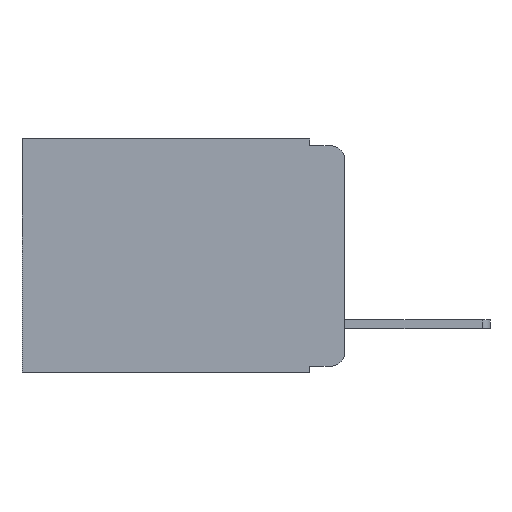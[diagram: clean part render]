
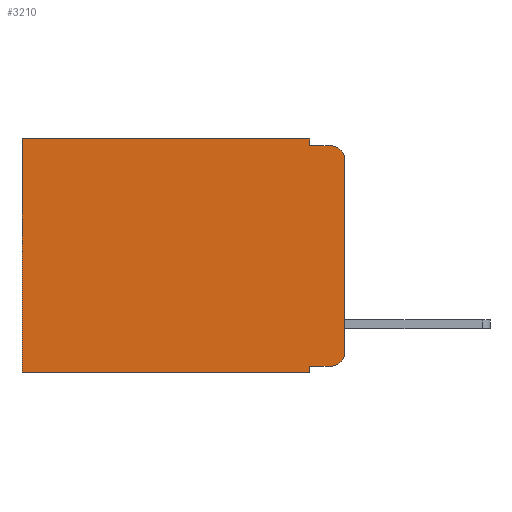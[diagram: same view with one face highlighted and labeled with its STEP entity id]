
A CAD part, left-side view. The second image highlights one B-rep face of the part: STEP entity #3210.
In plain terms, the highlighted planar face has unit normal (-1, 0, 0).
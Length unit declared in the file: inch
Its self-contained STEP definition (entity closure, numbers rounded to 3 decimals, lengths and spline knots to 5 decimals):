
#329 = ORIENTED_EDGE ( 'NONE', *, *, #6118, .T. ) ;
#747 = VERTEX_POINT ( 'NONE', #6597 ) ;
#798 = ORIENTED_EDGE ( 'NONE', *, *, #7005, .F. ) ;
#981 = DIRECTION ( 'NONE',  ( 0., 0., -1. ) ) ;
#1131 = LINE ( 'NONE', #3052, #11477 ) ;
#1171 = VERTEX_POINT ( 'NONE', #14665 ) ;
#1192 = DIRECTION ( 'NONE',  ( 0., 0., -1. ) ) ;
#1352 = DIRECTION ( 'NONE',  ( 0., 1., 0. ) ) ;
#1568 = VECTOR ( 'NONE', #981, 39.37008 ) ;
#1901 = VECTOR ( 'NONE', #5863, 39.37008 ) ;
#1966 = DIRECTION ( 'NONE',  ( -1., 0., 0. ) ) ;
#2011 = LINE ( 'NONE', #13183, #1568 ) ;
#2070 = DIRECTION ( 'NONE',  ( 0., -1., 0. ) ) ;
#2129 = CARTESIAN_POINT ( 'NONE',  ( 0.298, 0.02, -0.03 ) ) ;
#2144 = CARTESIAN_POINT ( 'NONE',  ( 0.298, 0.473, -0.343 ) ) ;
#2473 = VECTOR ( 'NONE', #2070, 39.37008 ) ;
#2561 = VERTEX_POINT ( 'NONE', #9913 ) ;
#2797 = DIRECTION ( 'NONE',  ( 0., -1., 0. ) ) ;
#3052 = CARTESIAN_POINT ( 'NONE',  ( 0.298, 0.051, 0. ) ) ;
#3210 = ADVANCED_FACE ( 'NONE', ( #14722 ), #9632, .F. ) ;
#3303 = CARTESIAN_POINT ( 'NONE',  ( 0.298, 0.02, -0.313 ) ) ;
#3344 = EDGE_CURVE ( 'NONE', #9361, #1171, #15693, .T. ) ;
#3514 = DIRECTION ( 'NONE',  ( 0., 0., -1. ) ) ;
#4251 = EDGE_CURVE ( 'NONE', #2561, #1171, #12303, .T. ) ;
#4436 = AXIS2_PLACEMENT_3D ( 'NONE', #2129, #1966, #3514 ) ;
#4647 = VERTEX_POINT ( 'NONE', #9723 ) ;
#4684 = DIRECTION ( 'NONE',  ( 0., 0., -1. ) ) ;
#5188 = EDGE_CURVE ( 'NONE', #12633, #2561, #1131, .T. ) ;
#5487 = VECTOR ( 'NONE', #7988, 39.37008 ) ;
#5863 = DIRECTION ( 'NONE',  ( 0., 0., -1. ) ) ;
#6118 = EDGE_CURVE ( 'NONE', #11728, #15267, #15860, .T. ) ;
#6186 = DIRECTION ( 'NONE',  ( 0., 0., -1. ) ) ;
#6189 = DIRECTION ( 'NONE',  ( 1., 0., 0. ) ) ;
#6198 = CARTESIAN_POINT ( 'NONE',  ( 0.298, 0.473, 0. ) ) ;
#6597 = CARTESIAN_POINT ( 'NONE',  ( 0.298, 0., -0.313 ) ) ;
#6918 = CARTESIAN_POINT ( 'NONE',  ( 0.298, 0.473, 0. ) ) ;
#7005 = EDGE_CURVE ( 'NONE', #10765, #13505, #2011, .T. ) ;
#7257 = ORIENTED_EDGE ( 'NONE', *, *, #5188, .F. ) ;
#7891 = LINE ( 'NONE', #10823, #14001 ) ;
#7988 = DIRECTION ( 'NONE',  ( 0., 0., -1. ) ) ;
#8004 = CARTESIAN_POINT ( 'NONE',  ( 0.298, 0., -0.03 ) ) ;
#8144 = DIRECTION ( 'NONE',  ( 0., 1., 0. ) ) ;
#8790 = EDGE_CURVE ( 'NONE', #10765, #4647, #7891, .T. ) ;
#9247 = VECTOR ( 'NONE', #1352, 39.37008 ) ;
#9361 = VERTEX_POINT ( 'NONE', #8004 ) ;
#9418 = AXIS2_PLACEMENT_3D ( 'NONE', #3303, #12614, #4684 ) ;
#9472 = CARTESIAN_POINT ( 'NONE',  ( 0.298, 0., -0.343 ) ) ;
#9632 = PLANE ( 'NONE',  #13619 ) ;
#9657 = EDGE_CURVE ( 'NONE', #4647, #747, #10943, .T. ) ;
#9723 = CARTESIAN_POINT ( 'NONE',  ( 0.298, 0.02, -0.333 ) ) ;
#9913 = CARTESIAN_POINT ( 'NONE',  ( 0.298, 0.051, -0.01 ) ) ;
#10765 = VERTEX_POINT ( 'NONE', #15559 ) ;
#10823 = CARTESIAN_POINT ( 'NONE',  ( 0.298, 0.051, -0.333 ) ) ;
#10943 = CIRCLE ( 'NONE', #9418, 0.02 ) ;
#11310 = CARTESIAN_POINT ( 'NONE',  ( 0.298, 0.051, -0.343 ) ) ;
#11334 = CARTESIAN_POINT ( 'NONE',  ( 0.298, 0.051, -0.01 ) ) ;
#11477 = VECTOR ( 'NONE', #1192, 39.37008 ) ;
#11728 = VERTEX_POINT ( 'NONE', #6198 ) ;
#12127 = CARTESIAN_POINT ( 'NONE',  ( 0.298, 0.051, 0. ) ) ;
#12303 = LINE ( 'NONE', #11334, #2473 ) ;
#12614 = DIRECTION ( 'NONE',  ( -1., 0., 0. ) ) ;
#12633 = VERTEX_POINT ( 'NONE', #12127 ) ;
#12708 = LINE ( 'NONE', #9472, #9247 ) ;
#12886 = VECTOR ( 'NONE', #8144, 39.37008 ) ;
#13183 = CARTESIAN_POINT ( 'NONE',  ( 0.298, 0.051, 0. ) ) ;
#13288 = LINE ( 'NONE', #14589, #12886 ) ;
#13355 = ORIENTED_EDGE ( 'NONE', *, *, #13443, .F. ) ;
#13443 = EDGE_CURVE ( 'NONE', #9361, #747, #15927, .T. ) ;
#13505 = VERTEX_POINT ( 'NONE', #11310 ) ;
#13619 = AXIS2_PLACEMENT_3D ( 'NONE', #14271, #6189, #6186 ) ;
#13657 = EDGE_LOOP ( 'NONE', ( #13355, #13749, #17115, #7257, #14160, #329, #14554, #798, #14959, #15729 ) ) ;
#13749 = ORIENTED_EDGE ( 'NONE', *, *, #3344, .T. ) ;
#13754 = CARTESIAN_POINT ( 'NONE',  ( 0.298, 0., 0. ) ) ;
#14001 = VECTOR ( 'NONE', #2797, 39.37008 ) ;
#14160 = ORIENTED_EDGE ( 'NONE', *, *, #15499, .T. ) ;
#14271 = CARTESIAN_POINT ( 'NONE',  ( 0.298, 0., 0. ) ) ;
#14554 = ORIENTED_EDGE ( 'NONE', *, *, #14944, .F. ) ;
#14589 = CARTESIAN_POINT ( 'NONE',  ( 0.298, 0., 0. ) ) ;
#14665 = CARTESIAN_POINT ( 'NONE',  ( 0.298, 0.02, -0.01 ) ) ;
#14722 = FACE_OUTER_BOUND ( 'NONE', #13657, .T. ) ;
#14944 = EDGE_CURVE ( 'NONE', #13505, #15267, #12708, .T. ) ;
#14959 = ORIENTED_EDGE ( 'NONE', *, *, #8790, .T. ) ;
#15267 = VERTEX_POINT ( 'NONE', #2144 ) ;
#15499 = EDGE_CURVE ( 'NONE', #12633, #11728, #13288, .T. ) ;
#15559 = CARTESIAN_POINT ( 'NONE',  ( 0.298, 0.051, -0.333 ) ) ;
#15693 = CIRCLE ( 'NONE', #4436, 0.02 ) ;
#15729 = ORIENTED_EDGE ( 'NONE', *, *, #9657, .T. ) ;
#15860 = LINE ( 'NONE', #6918, #5487 ) ;
#15927 = LINE ( 'NONE', #13754, #1901 ) ;
#17115 = ORIENTED_EDGE ( 'NONE', *, *, #4251, .F. ) ;
